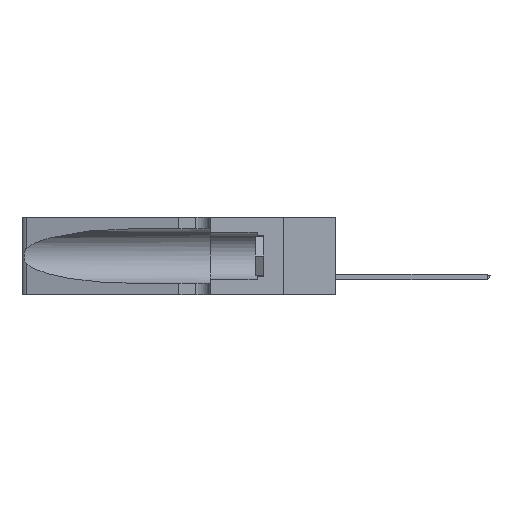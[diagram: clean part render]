
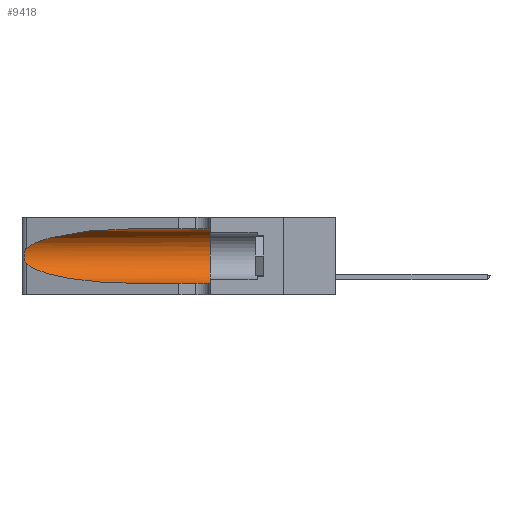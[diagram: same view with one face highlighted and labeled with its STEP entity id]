
A CAD part, left-side view. The second image highlights one B-rep face of the part: STEP entity #9418.
In plain terms, the highlighted cylindrical face has radius 3.308 mm (diameter 6.617 mm), a partial arc.
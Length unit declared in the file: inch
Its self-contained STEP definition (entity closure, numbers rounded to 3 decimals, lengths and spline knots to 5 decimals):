
#689 = VERTEX_POINT ( 'NONE', #24000 ) ;
#1307 = DIRECTION ( 'NONE',  ( 0., 1., 0. ) ) ;
#2373 = CARTESIAN_POINT ( 'NONE',  ( 0.25787, 1.23484, 0.2124 ) ) ;
#2996 = CARTESIAN_POINT ( 'NONE',  ( 0.1305, 0.72297, 0.31525 ) ) ;
#3579 = CARTESIAN_POINT ( 'NONE',  ( 0.25487, 1.22718, 0.14631 ) ) ;
#3742 =( BOUNDED_CURVE ( )  B_SPLINE_CURVE ( 3, ( #3579, #6012, #20507, #23843 ),
 .UNSPECIFIED., .F., .T. ) 
 B_SPLINE_CURVE_WITH_KNOTS ( ( 4, 4 ),
 ( 3.44316, 4.71239 ),
 .UNSPECIFIED. ) 
 CURVE ( )  GEOMETRIC_REPRESENTATION_ITEM ( )  RATIONAL_B_SPLINE_CURVE ( ( 1., 0.87, 0.87, 1. ) ) 
 REPRESENTATION_ITEM ( '' )  );
#3945 = CARTESIAN_POINT ( 'NONE',  ( 0.1305, 0.72297, 0.05475 ) ) ;
#4130 = VERTEX_POINT ( 'NONE', #31199 ) ;
#4472 = EDGE_CURVE ( 'NONE', #36205, #26711, #33146, .T. ) ;
#5056 = CARTESIAN_POINT ( 'NONE',  ( 0.1305, 0.35, 0.05475 ) ) ;
#5070 = VECTOR ( 'NONE', #10039, 39.37008 ) ;
#5408 = CARTESIAN_POINT ( 'NONE',  ( 0.25487, 1.22718, 0.14631 ) ) ;
#5790 = CARTESIAN_POINT ( 'NONE',  ( 0.18966, 0.96281, 0.31525 ) ) ;
#5944 = VERTEX_POINT ( 'NONE', #5056 ) ;
#6012 = CARTESIAN_POINT ( 'NONE',  ( 0.2373, 1.15595, 0.08982 ) ) ;
#6807 = CARTESIAN_POINT ( 'NONE',  ( 0.1305, 1.61858, 0.31525 ) ) ;
#7642 = CARTESIAN_POINT ( 'NONE',  ( 0.25487, 1.22718, 0.22369 ) ) ;
#8856 = CARTESIAN_POINT ( 'NONE',  ( 0.2373, 1.15595, 0.28018 ) ) ;
#9418 = ADVANCED_FACE ( 'NONE', ( #14786 ), #13954, .F. ) ;
#9919 = CARTESIAN_POINT ( 'NONE',  ( 0.1305, 1.61858, 0.05475 ) ) ;
#10039 = DIRECTION ( 'NONE',  ( 0., -1., 0. ) ) ;
#10043 = AXIS2_PLACEMENT_3D ( 'NONE', #15297, #1307, #21196 ) ;
#10336 =( BOUNDED_CURVE ( )  B_SPLINE_CURVE ( 3, ( #2996, #5790, #8856, #17669 ),
 .UNSPECIFIED., .F., .T. ) 
 B_SPLINE_CURVE_WITH_KNOTS ( ( 4, 4 ),
 ( 1.5708, 2.84003 ),
 .UNSPECIFIED. ) 
 CURVE ( )  GEOMETRIC_REPRESENTATION_ITEM ( )  RATIONAL_B_SPLINE_CURVE ( ( 1., 0.87, 0.87, 1. ) ) 
 REPRESENTATION_ITEM ( '' )  );
#10875 = CARTESIAN_POINT ( 'NONE',  ( 0.26075, 1.23896, 0.178 ) ) ;
#11317 = CARTESIAN_POINT ( 'NONE',  ( 0.25789, 1.23486, 0.15765 ) ) ;
#12241 = DIRECTION ( 'NONE',  ( 0., -1., 0. ) ) ;
#12515 = ORIENTED_EDGE ( 'NONE', *, *, #4472, .T. ) ;
#13908 = CARTESIAN_POINT ( 'NONE',  ( 0.25856, 1.23593, 0.16098 ) ) ;
#13954 = CYLINDRICAL_SURFACE ( 'NONE', #20302, 0.13025 ) ;
#14786 = FACE_OUTER_BOUND ( 'NONE', #23573, .T. ) ;
#15297 = CARTESIAN_POINT ( 'NONE',  ( 0.1305, 0.35, 0.185 ) ) ;
#16214 = CARTESIAN_POINT ( 'NONE',  ( 0.25854, 1.2359, 0.20912 ) ) ;
#16572 = DIRECTION ( 'NONE',  ( 0., 0., -1. ) ) ;
#17502 = ORIENTED_EDGE ( 'NONE', *, *, #19023, .T. ) ;
#17669 = CARTESIAN_POINT ( 'NONE',  ( 0.25487, 1.22718, 0.22369 ) ) ;
#18983 = CARTESIAN_POINT ( 'NONE',  ( 0.25487, 1.22718, 0.14631 ) ) ;
#19023 = EDGE_CURVE ( 'NONE', #4130, #36205, #10336, .T. ) ;
#19041 = CARTESIAN_POINT ( 'NONE',  ( 0.26018, 1.23835, 0.19895 ) ) ;
#19118 = LINE ( 'NONE', #9919, #5070 ) ;
#20302 = AXIS2_PLACEMENT_3D ( 'NONE', #33308, #24801, #16572 ) ;
#20507 = CARTESIAN_POINT ( 'NONE',  ( 0.18966, 0.96281, 0.05475 ) ) ;
#21196 = DIRECTION ( 'NONE',  ( 0., 0., 1. ) ) ;
#21653 = ORIENTED_EDGE ( 'NONE', *, *, #34051, .T. ) ;
#22548 = CARTESIAN_POINT ( 'NONE',  ( 0.25555, 1.22993, 0.14849 ) ) ;
#23093 = CIRCLE ( 'NONE', #10043, 0.13025 ) ;
#23573 = EDGE_LOOP ( 'NONE', ( #17502, #12515, #30594, #21653, #35602, #30345 ) ) ;
#23821 = LINE ( 'NONE', #6807, #33416 ) ;
#23843 = CARTESIAN_POINT ( 'NONE',  ( 0.1305, 0.72297, 0.05475 ) ) ;
#24000 = CARTESIAN_POINT ( 'NONE',  ( 0.1305, 0.35, 0.31525 ) ) ;
#24246 = EDGE_CURVE ( 'NONE', #689, #5944, #23093, .T. ) ;
#24784 = EDGE_CURVE ( 'NONE', #26711, #32834, #3742, .T. ) ;
#24801 = DIRECTION ( 'NONE',  ( 0., -1., 0. ) ) ;
#26711 = VERTEX_POINT ( 'NONE', #18983 ) ;
#27597 = CARTESIAN_POINT ( 'NONE',  ( 0.26075, 1.23896, 0.19203 ) ) ;
#29368 = CARTESIAN_POINT ( 'NONE',  ( 0.25487, 1.22718, 0.22369 ) ) ;
#29741 = EDGE_CURVE ( 'NONE', #4130, #689, #23821, .T. ) ;
#30270 = CARTESIAN_POINT ( 'NONE',  ( 0.25555, 1.22994, 0.2215 ) ) ;
#30345 = ORIENTED_EDGE ( 'NONE', *, *, #29741, .F. ) ;
#30594 = ORIENTED_EDGE ( 'NONE', *, *, #24784, .T. ) ;
#31199 = CARTESIAN_POINT ( 'NONE',  ( 0.1305, 0.72297, 0.31525 ) ) ;
#32834 = VERTEX_POINT ( 'NONE', #3945 ) ;
#32937 = CARTESIAN_POINT ( 'NONE',  ( 0.25639, 1.23184, 0.21858 ) ) ;
#33146 = B_SPLINE_CURVE_WITH_KNOTS ( 'NONE', 3,
 ( #7642, #30270, #32937, #2373, #16214, #19041, #27597, #10875, #36024, #13908, #11317, #33411, #22548, #5408 ),
 .UNSPECIFIED., .F., .F.,
 ( 4, 2, 2, 2, 2, 2, 4 ),
 ( 0., 0.00027, 0.00053, 0.00107, 0.0016, 0.00187, 0.00214 ),
 .UNSPECIFIED. ) ;
#33308 = CARTESIAN_POINT ( 'NONE',  ( 0.1305, 1.61858, 0.185 ) ) ;
#33411 = CARTESIAN_POINT ( 'NONE',  ( 0.25639, 1.23186, 0.15144 ) ) ;
#33416 = VECTOR ( 'NONE', #12241, 39.37008 ) ;
#34051 = EDGE_CURVE ( 'NONE', #32834, #5944, #19118, .T. ) ;
#35602 = ORIENTED_EDGE ( 'NONE', *, *, #24246, .F. ) ;
#36024 = CARTESIAN_POINT ( 'NONE',  ( 0.26017, 1.23833, 0.17102 ) ) ;
#36205 = VERTEX_POINT ( 'NONE', #29368 ) ;
